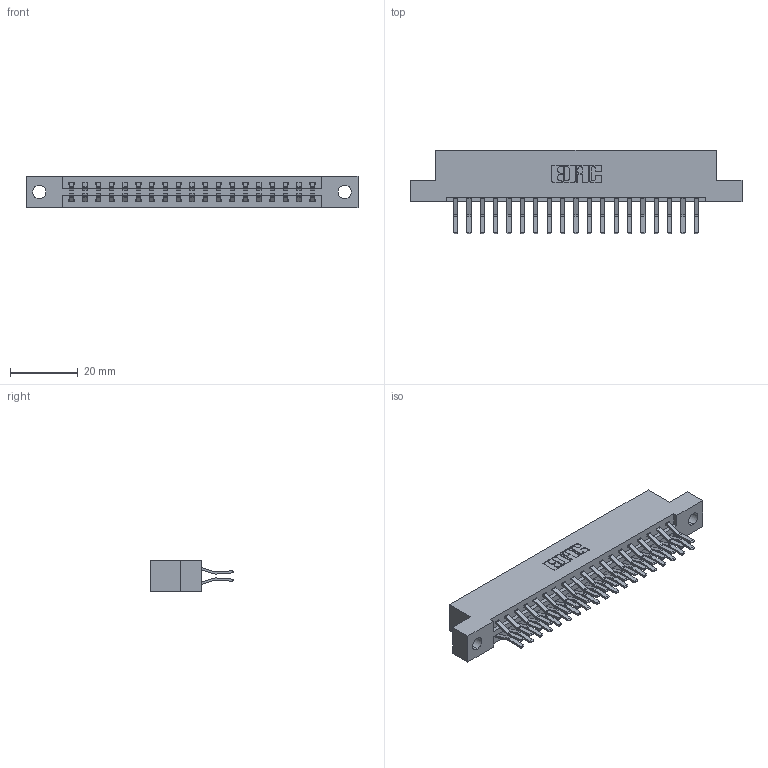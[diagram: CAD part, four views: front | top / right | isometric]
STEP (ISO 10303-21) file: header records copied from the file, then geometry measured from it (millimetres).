
FILE_DESCRIPTION (( 'STEP AP203' ), '1' );
FILE_NAME ('337-038-560-204.STEP', '2018-08-08T06:18:19', ( '' ), ( '' ), 'SwSTEP 2.0', 'SolidWorks 2016', '' );
FILE_SCHEMA (( 'CONFIG_CONTROL_DESIGN' ));
Length unit declared in the file: inch
Products named in the file (3): 337 Part_Flush Mounting Lugs - 0.156 Dia-TH; 345-292-001_560 Tail; 337-038-560-204
Assembly tree (39 placements, depth 2):
  337-038-560-204
    337 Part_Flush Mounting Lugs - 0.156 Dia-TH
    345-292-001_560 Tail  x38
Bounding box: 98.3 x 24.78 x 9.4 mm (x, y, z)
Volume: 10214.5 mm3; surface area: 11842.4 mm2
Topology: 39 solids, 39 shells, 2242 faces, 6657 edges, 4386 vertices
Faces by surface type: plane 1514, cylinder 728
Entity records: 17797 total; most frequent: CARTESIAN_POINT 3018, ORIENTED_EDGE 2954, DIRECTION 2613, EDGE_CURVE 1477, VECTOR 1345, LINE 1345, VERTEX_POINT 982, AXIS2_PLACEMENT_3D 634
